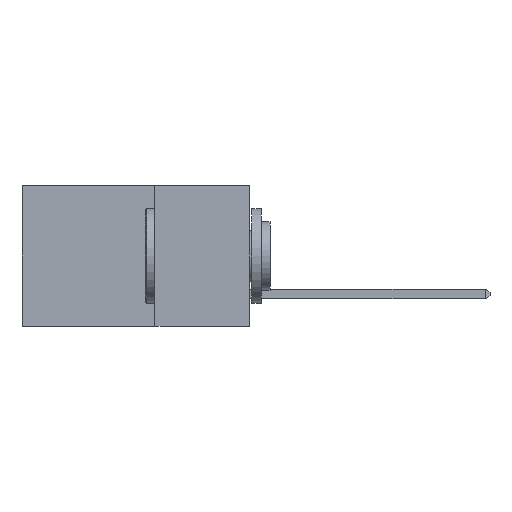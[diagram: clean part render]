
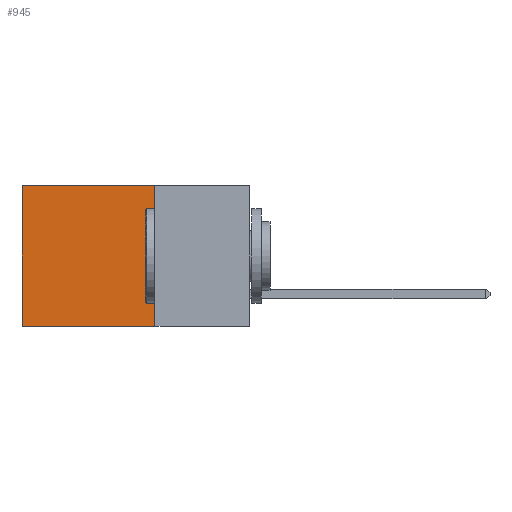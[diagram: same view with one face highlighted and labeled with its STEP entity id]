
A CAD part, left-side view. The second image highlights one B-rep face of the part: STEP entity #945.
In plain terms, the highlighted planar face has unit normal (-1, 0, 0).
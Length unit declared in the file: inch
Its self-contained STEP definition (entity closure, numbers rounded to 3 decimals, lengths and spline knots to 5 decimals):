
#226 = DIRECTION ( 'NONE',  ( 1., 0., 0. ) ) ;
#455 = CARTESIAN_POINT ( 'NONE',  ( 0.2875, 0.6, 0. ) ) ;
#945 = ADVANCED_FACE ( 'NONE', ( #10407 ), #14028, .F. ) ;
#1110 = CARTESIAN_POINT ( 'NONE',  ( 0.2875, 0.25, 0. ) ) ;
#1622 = VERTEX_POINT ( 'NONE', #455 ) ;
#2264 = CARTESIAN_POINT ( 'NONE',  ( 0.2875, 0.25, 0. ) ) ;
#2882 = DIRECTION ( 'NONE',  ( 0., 1., 0. ) ) ;
#3500 = ORIENTED_EDGE ( 'NONE', *, *, #14505, .T. ) ;
#3942 = VERTEX_POINT ( 'NONE', #2264 ) ;
#4678 = ORIENTED_EDGE ( 'NONE', *, *, #18256, .T. ) ;
#5148 = VECTOR ( 'NONE', #19998, 39.37008 ) ;
#5483 = LINE ( 'NONE', #1110, #13365 ) ;
#5526 = VECTOR ( 'NONE', #12248, 39.37008 ) ;
#5961 = CARTESIAN_POINT ( 'NONE',  ( 0.2875, 0.25, -0.37 ) ) ;
#6690 = CARTESIAN_POINT ( 'NONE',  ( 0.2875, 0.6, 0. ) ) ;
#6894 = ORIENTED_EDGE ( 'NONE', *, *, #16584, .F. ) ;
#9321 = CARTESIAN_POINT ( 'NONE',  ( 0.2875, 0.25, 0. ) ) ;
#10310 = VERTEX_POINT ( 'NONE', #14499 ) ;
#10407 = FACE_OUTER_BOUND ( 'NONE', #19479, .T. ) ;
#10787 = CARTESIAN_POINT ( 'NONE',  ( 0.2875, 0.25, 0. ) ) ;
#11058 = LINE ( 'NONE', #6690, #20056 ) ;
#12248 = DIRECTION ( 'NONE',  ( 0., 1., 0. ) ) ;
#13055 = LINE ( 'NONE', #9321, #5148 ) ;
#13365 = VECTOR ( 'NONE', #2882, 39.37008 ) ;
#13745 = EDGE_CURVE ( 'NONE', #16940, #10310, #17396, .T. ) ;
#14028 = PLANE ( 'NONE',  #20141 ) ;
#14499 = CARTESIAN_POINT ( 'NONE',  ( 0.2875, 0.6, -0.37 ) ) ;
#14505 = EDGE_CURVE ( 'NONE', #3942, #1622, #5483, .T. ) ;
#14541 = DIRECTION ( 'NONE',  ( 0., 0., -1. ) ) ;
#15064 = CARTESIAN_POINT ( 'NONE',  ( 0.2875, 0.25, -0.37 ) ) ;
#16584 = EDGE_CURVE ( 'NONE', #3942, #16940, #13055, .T. ) ;
#16940 = VERTEX_POINT ( 'NONE', #15064 ) ;
#17396 = LINE ( 'NONE', #5961, #5526 ) ;
#18256 = EDGE_CURVE ( 'NONE', #1622, #10310, #11058, .T. ) ;
#19295 = DIRECTION ( 'NONE',  ( 0., 0., -1. ) ) ;
#19479 = EDGE_LOOP ( 'NONE', ( #4678, #19715, #6894, #3500 ) ) ;
#19715 = ORIENTED_EDGE ( 'NONE', *, *, #13745, .F. ) ;
#19998 = DIRECTION ( 'NONE',  ( 0., 0., -1. ) ) ;
#20056 = VECTOR ( 'NONE', #14541, 39.37008 ) ;
#20141 = AXIS2_PLACEMENT_3D ( 'NONE', #10787, #226, #19295 ) ;
